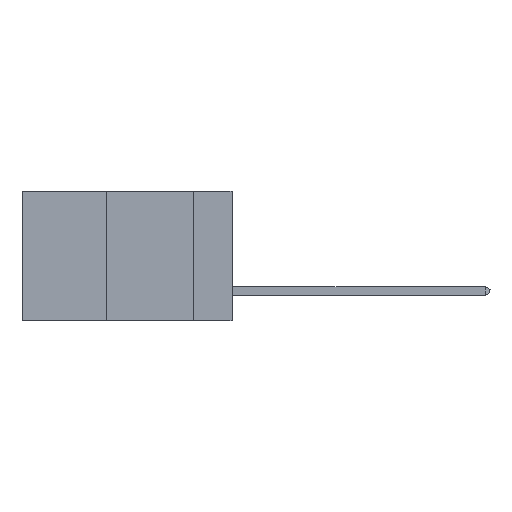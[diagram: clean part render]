
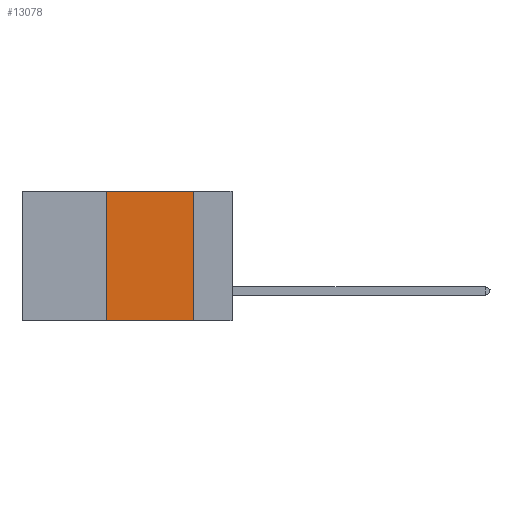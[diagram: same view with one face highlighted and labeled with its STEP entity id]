
A CAD part, left-side view. The second image highlights one B-rep face of the part: STEP entity #13078.
In plain terms, the highlighted planar face has unit normal (-1, 0, 0).
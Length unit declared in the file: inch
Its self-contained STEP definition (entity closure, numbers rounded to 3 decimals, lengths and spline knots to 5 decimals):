
#3142 = ORIENTED_EDGE ( 'NONE', *, *, #24660, .F. ) ;
#3773 = CARTESIAN_POINT ( 'NONE',  ( 0., 0.11, 0. ) ) ;
#3989 = DIRECTION ( 'NONE',  ( 0., -1., 0. ) ) ;
#4263 = DIRECTION ( 'NONE',  ( 0., 0., -1. ) ) ;
#4647 = CARTESIAN_POINT ( 'NONE',  ( 0., 0.36, 0. ) ) ;
#4847 = LINE ( 'NONE', #16419, #7187 ) ;
#5155 = VERTEX_POINT ( 'NONE', #10169 ) ;
#5801 = EDGE_CURVE ( 'NONE', #11365, #22312, #6317, .T. ) ;
#6317 = LINE ( 'NONE', #22550, #19824 ) ;
#6497 = CARTESIAN_POINT ( 'NONE',  ( 0., 0.6, 0. ) ) ;
#6882 = VECTOR ( 'NONE', #3989, 39.37008 ) ;
#7187 = VECTOR ( 'NONE', #14509, 39.37008 ) ;
#7444 = EDGE_CURVE ( 'NONE', #5155, #22312, #26315, .T. ) ;
#7856 = VERTEX_POINT ( 'NONE', #4647 ) ;
#8459 = ORIENTED_EDGE ( 'NONE', *, *, #9896, .F. ) ;
#9896 = EDGE_CURVE ( 'NONE', #7856, #11365, #11399, .T. ) ;
#9941 = FACE_OUTER_BOUND ( 'NONE', #17166, .T. ) ;
#10169 = CARTESIAN_POINT ( 'NONE',  ( 0., 0.36, -0.37 ) ) ;
#11045 = VECTOR ( 'NONE', #15825, 39.37008 ) ;
#11365 = VERTEX_POINT ( 'NONE', #3773 ) ;
#11399 = LINE ( 'NONE', #18119, #11045 ) ;
#13078 = ADVANCED_FACE ( 'NONE', ( #9941 ), #25482, .F. ) ;
#13901 = AXIS2_PLACEMENT_3D ( 'NONE', #6497, #19043, #23259 ) ;
#14509 = DIRECTION ( 'NONE',  ( 0., 0., 1. ) ) ;
#15825 = DIRECTION ( 'NONE',  ( 0., -1., 0. ) ) ;
#16419 = CARTESIAN_POINT ( 'NONE',  ( 0., 0.36, 0. ) ) ;
#17166 = EDGE_LOOP ( 'NONE', ( #26240, #8459, #3142, #17851 ) ) ;
#17851 = ORIENTED_EDGE ( 'NONE', *, *, #7444, .T. ) ;
#18119 = CARTESIAN_POINT ( 'NONE',  ( 0., 0.6, 0. ) ) ;
#19043 = DIRECTION ( 'NONE',  ( 1., 0., 0. ) ) ;
#19824 = VECTOR ( 'NONE', #4263, 39.37008 ) ;
#21357 = CARTESIAN_POINT ( 'NONE',  ( 0., 0.11, -0.37 ) ) ;
#22312 = VERTEX_POINT ( 'NONE', #21357 ) ;
#22550 = CARTESIAN_POINT ( 'NONE',  ( 0., 0.11, 0. ) ) ;
#23259 = DIRECTION ( 'NONE',  ( 0., 0., -1. ) ) ;
#24660 = EDGE_CURVE ( 'NONE', #5155, #7856, #4847, .T. ) ;
#24674 = CARTESIAN_POINT ( 'NONE',  ( 0., 0.6, -0.37 ) ) ;
#25482 = PLANE ( 'NONE',  #13901 ) ;
#26240 = ORIENTED_EDGE ( 'NONE', *, *, #5801, .F. ) ;
#26315 = LINE ( 'NONE', #24674, #6882 ) ;
